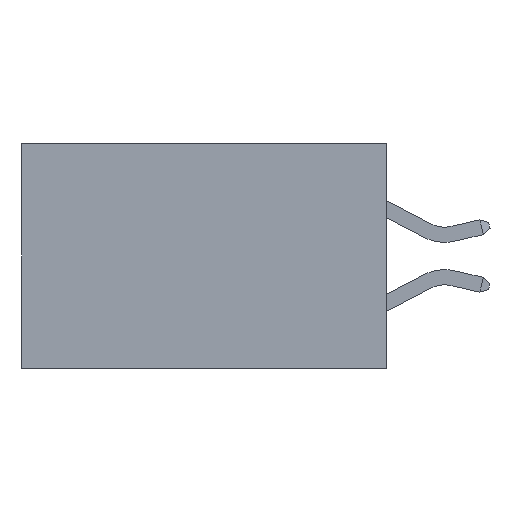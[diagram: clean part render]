
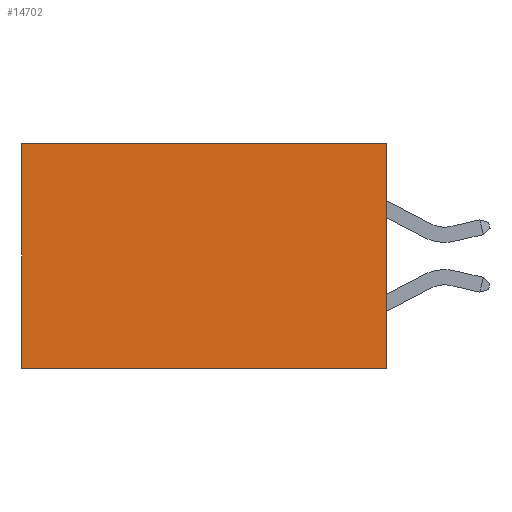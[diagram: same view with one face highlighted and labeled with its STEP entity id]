
A CAD part, left-side view. The second image highlights one B-rep face of the part: STEP entity #14702.
In plain terms, the highlighted planar face has unit normal (-1, 0, 0).
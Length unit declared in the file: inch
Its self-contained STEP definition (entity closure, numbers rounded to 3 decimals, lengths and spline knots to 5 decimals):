
#1405 = LINE ( 'NONE', #9479, #8343 ) ;
#3853 = VERTEX_POINT ( 'NONE', #30502 ) ;
#4733 = DIRECTION ( 'NONE',  ( 0., 0., -1. ) ) ;
#5198 = VECTOR ( 'NONE', #23717, 39.37008 ) ;
#5574 = CARTESIAN_POINT ( 'NONE',  ( 0.298, 0., 0. ) ) ;
#6036 = LINE ( 'NONE', #21207, #5198 ) ;
#7229 = FACE_OUTER_BOUND ( 'NONE', #8139, .T. ) ;
#7566 = LINE ( 'NONE', #15593, #27111 ) ;
#7847 = ORIENTED_EDGE ( 'NONE', *, *, #16248, .F. ) ;
#8139 = EDGE_LOOP ( 'NONE', ( #28857, #23111, #7847, #21719 ) ) ;
#8343 = VECTOR ( 'NONE', #22327, 39.37008 ) ;
#9280 = EDGE_CURVE ( 'NONE', #3853, #17851, #7566, .T. ) ;
#9479 = CARTESIAN_POINT ( 'NONE',  ( 0.298, 0.6, 0. ) ) ;
#9557 = VERTEX_POINT ( 'NONE', #11376 ) ;
#11376 = CARTESIAN_POINT ( 'NONE',  ( 0.298, 0., 0. ) ) ;
#12991 = DIRECTION ( 'NONE',  ( 0., 1., 0. ) ) ;
#13576 = DIRECTION ( 'NONE',  ( 0., 1., 0. ) ) ;
#14702 = ADVANCED_FACE ( 'NONE', ( #7229 ), #32767, .F. ) ;
#15126 = VERTEX_POINT ( 'NONE', #19050 ) ;
#15593 = CARTESIAN_POINT ( 'NONE',  ( 0.298, 0., -0.37 ) ) ;
#16248 = EDGE_CURVE ( 'NONE', #9557, #3853, #6036, .T. ) ;
#17464 = AXIS2_PLACEMENT_3D ( 'NONE', #17662, #20167, #4733 ) ;
#17662 = CARTESIAN_POINT ( 'NONE',  ( 0.298, 0., 0. ) ) ;
#17851 = VERTEX_POINT ( 'NONE', #19577 ) ;
#17905 = EDGE_CURVE ( 'NONE', #15126, #17851, #1405, .T. ) ;
#19050 = CARTESIAN_POINT ( 'NONE',  ( 0.298, 0.6, 0. ) ) ;
#19577 = CARTESIAN_POINT ( 'NONE',  ( 0.298, 0.6, -0.37 ) ) ;
#20145 = LINE ( 'NONE', #5574, #26849 ) ;
#20167 = DIRECTION ( 'NONE',  ( 1., 0., 0. ) ) ;
#21207 = CARTESIAN_POINT ( 'NONE',  ( 0.298, 0., 0. ) ) ;
#21719 = ORIENTED_EDGE ( 'NONE', *, *, #29909, .T. ) ;
#22327 = DIRECTION ( 'NONE',  ( 0., 0., -1. ) ) ;
#23111 = ORIENTED_EDGE ( 'NONE', *, *, #9280, .F. ) ;
#23717 = DIRECTION ( 'NONE',  ( 0., 0., -1. ) ) ;
#26849 = VECTOR ( 'NONE', #13576, 39.37008 ) ;
#27111 = VECTOR ( 'NONE', #12991, 39.37008 ) ;
#28857 = ORIENTED_EDGE ( 'NONE', *, *, #17905, .T. ) ;
#29909 = EDGE_CURVE ( 'NONE', #9557, #15126, #20145, .T. ) ;
#30502 = CARTESIAN_POINT ( 'NONE',  ( 0.298, 0., -0.37 ) ) ;
#32767 = PLANE ( 'NONE',  #17464 ) ;
